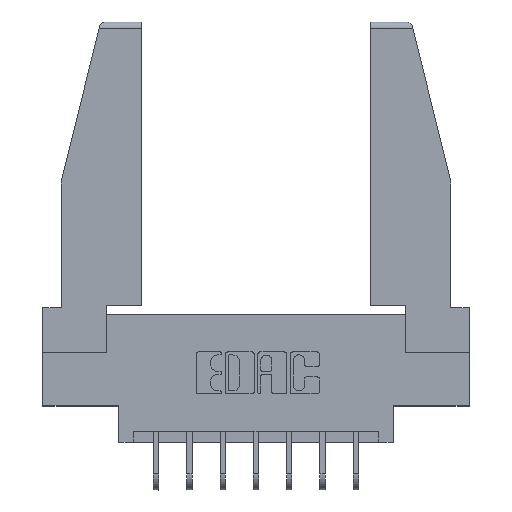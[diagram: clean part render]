
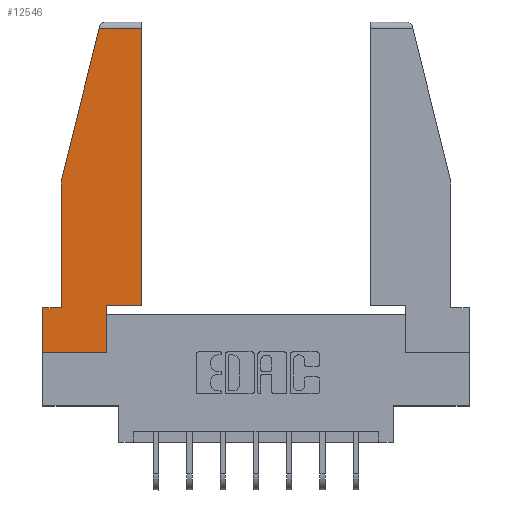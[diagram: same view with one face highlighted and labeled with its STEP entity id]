
A CAD part, top view. The second image highlights one B-rep face of the part: STEP entity #12546.
In plain terms, the highlighted planar face has unit normal (0, 0, 1).
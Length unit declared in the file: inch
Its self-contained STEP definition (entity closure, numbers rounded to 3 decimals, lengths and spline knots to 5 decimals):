
#383 = DIRECTION ( 'NONE',  ( 1., 0., 0. ) ) ;
#563 = EDGE_CURVE ( 'NONE', #823, #4381, #2620, .T. ) ;
#823 = VERTEX_POINT ( 'NONE', #4366 ) ;
#836 = EDGE_CURVE ( 'NONE', #4381, #5130, #9013, .T. ) ;
#992 = VERTEX_POINT ( 'NONE', #12483 ) ;
#1129 = CARTESIAN_POINT ( 'NONE',  ( 0., 0., 0. ) ) ;
#1362 = VECTOR ( 'NONE', #1543, 39.37008 ) ;
#1543 = DIRECTION ( 'NONE',  ( 1., 0., 0. ) ) ;
#1646 = LINE ( 'NONE', #7666, #7742 ) ;
#2142 = PLANE ( 'NONE',  #7419 ) ;
#2402 = EDGE_LOOP ( 'NONE', ( #7695, #10651, #10674, #13068, #13719, #4190, #2836, #6090, #7486 ) ) ;
#2405 = LINE ( 'NONE', #6061, #1362 ) ;
#2620 = LINE ( 'NONE', #3773, #4513 ) ;
#2835 = EDGE_CURVE ( 'NONE', #11119, #4960, #5666, .T. ) ;
#2836 = ORIENTED_EDGE ( 'NONE', *, *, #10783, .T. ) ;
#2861 = LINE ( 'NONE', #6163, #11702 ) ;
#3339 = DIRECTION ( 'NONE',  ( 0., 0., 1. ) ) ;
#3590 = VECTOR ( 'NONE', #9658, 39.37008 ) ;
#3605 = LINE ( 'NONE', #4553, #7625 ) ;
#3670 = CARTESIAN_POINT ( 'NONE',  ( 0.2636, 1.52, 0. ) ) ;
#3773 = CARTESIAN_POINT ( 'NONE',  ( 0.297, 0.223, 0. ) ) ;
#3855 = DIRECTION ( 'NONE',  ( 0., -1., 0. ) ) ;
#3898 = LINE ( 'NONE', #4134, #10307 ) ;
#4134 = CARTESIAN_POINT ( 'NONE',  ( 0., 1.52, 0. ) ) ;
#4190 = ORIENTED_EDGE ( 'NONE', *, *, #9982, .T. ) ;
#4366 = CARTESIAN_POINT ( 'NONE',  ( 0.297, 0.223, 0. ) ) ;
#4381 = VERTEX_POINT ( 'NONE', #10336 ) ;
#4400 = DIRECTION ( 'NONE',  ( 1., 0., 0. ) ) ;
#4457 = CARTESIAN_POINT ( 'NONE',  ( 0.297, 0., 0. ) ) ;
#4513 = VECTOR ( 'NONE', #383, 39.37008 ) ;
#4553 = CARTESIAN_POINT ( 'NONE',  ( 0.297, 0., 0. ) ) ;
#4960 = VERTEX_POINT ( 'NONE', #13626 ) ;
#4966 = VECTOR ( 'NONE', #9912, 39.37008 ) ;
#5130 = VERTEX_POINT ( 'NONE', #8609 ) ;
#5666 = LINE ( 'NONE', #9717, #4966 ) ;
#5828 = EDGE_CURVE ( 'NONE', #5130, #11119, #3898, .T. ) ;
#5918 = VECTOR ( 'NONE', #7656, 39.37008 ) ;
#6061 = CARTESIAN_POINT ( 'NONE',  ( 0., 0., 0. ) ) ;
#6090 = ORIENTED_EDGE ( 'NONE', *, *, #7443, .T. ) ;
#6163 = CARTESIAN_POINT ( 'NONE',  ( 0., 0.21, 0. ) ) ;
#6717 = DIRECTION ( 'NONE',  ( 0., 1., 0. ) ) ;
#7063 = CARTESIAN_POINT ( 'NONE',  ( 0., 0.21, 0. ) ) ;
#7419 = AXIS2_PLACEMENT_3D ( 'NONE', #1129, #3339, #4400 ) ;
#7443 = EDGE_CURVE ( 'NONE', #9158, #823, #3605, .T. ) ;
#7486 = ORIENTED_EDGE ( 'NONE', *, *, #563, .T. ) ;
#7625 = VECTOR ( 'NONE', #6717, 39.37008 ) ;
#7656 = DIRECTION ( 'NONE',  ( 0., 1., 0. ) ) ;
#7666 = CARTESIAN_POINT ( 'NONE',  ( 0., 0.21, 0. ) ) ;
#7695 = ORIENTED_EDGE ( 'NONE', *, *, #836, .T. ) ;
#7742 = VECTOR ( 'NONE', #8810, 39.37008 ) ;
#8573 = DIRECTION ( 'NONE',  ( -1., 0., 0. ) ) ;
#8609 = CARTESIAN_POINT ( 'NONE',  ( 0.461, 1.52, 0. ) ) ;
#8810 = DIRECTION ( 'NONE',  ( -1., 0., 0. ) ) ;
#8882 = VERTEX_POINT ( 'NONE', #7063 ) ;
#9013 = LINE ( 'NONE', #13178, #5918 ) ;
#9158 = VERTEX_POINT ( 'NONE', #4457 ) ;
#9443 = EDGE_CURVE ( 'NONE', #10796, #8882, #1646, .T. ) ;
#9658 = DIRECTION ( 'NONE',  ( 0., -1., 0. ) ) ;
#9717 = CARTESIAN_POINT ( 'NONE',  ( 0.271, 1.55, 0. ) ) ;
#9912 = DIRECTION ( 'NONE',  ( -0.239, -0.971, 0. ) ) ;
#9982 = EDGE_CURVE ( 'NONE', #8882, #992, #2861, .T. ) ;
#10307 = VECTOR ( 'NONE', #8573, 39.37008 ) ;
#10336 = CARTESIAN_POINT ( 'NONE',  ( 0.461, 0.223, 0. ) ) ;
#10465 = FACE_OUTER_BOUND ( 'NONE', #2402, .T. ) ;
#10634 = CARTESIAN_POINT ( 'NONE',  ( 0.086, 0.8, 0. ) ) ;
#10651 = ORIENTED_EDGE ( 'NONE', *, *, #5828, .T. ) ;
#10674 = ORIENTED_EDGE ( 'NONE', *, *, #2835, .T. ) ;
#10783 = EDGE_CURVE ( 'NONE', #992, #9158, #2405, .T. ) ;
#10796 = VERTEX_POINT ( 'NONE', #12785 ) ;
#11033 = EDGE_CURVE ( 'NONE', #4960, #10796, #13862, .T. ) ;
#11119 = VERTEX_POINT ( 'NONE', #3670 ) ;
#11702 = VECTOR ( 'NONE', #3855, 39.37008 ) ;
#12483 = CARTESIAN_POINT ( 'NONE',  ( 0., 0., 0. ) ) ;
#12546 = ADVANCED_FACE ( 'NONE', ( #10465 ), #2142, .T. ) ;
#12785 = CARTESIAN_POINT ( 'NONE',  ( 0.086, 0.21, 0. ) ) ;
#13068 = ORIENTED_EDGE ( 'NONE', *, *, #11033, .T. ) ;
#13178 = CARTESIAN_POINT ( 'NONE',  ( 0.461, 0.223, 0. ) ) ;
#13626 = CARTESIAN_POINT ( 'NONE',  ( 0.086, 0.8, 0. ) ) ;
#13719 = ORIENTED_EDGE ( 'NONE', *, *, #9443, .T. ) ;
#13862 = LINE ( 'NONE', #10634, #3590 ) ;
